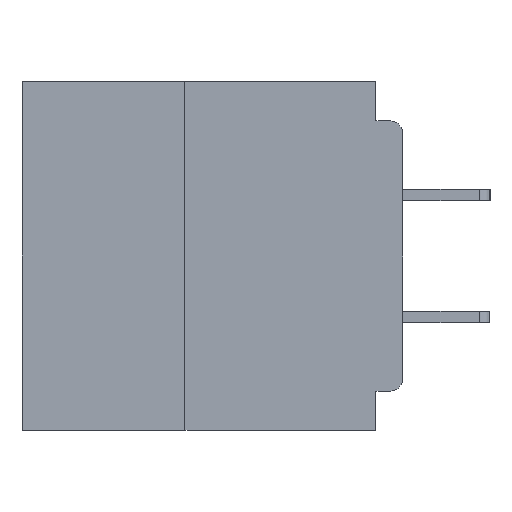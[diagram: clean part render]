
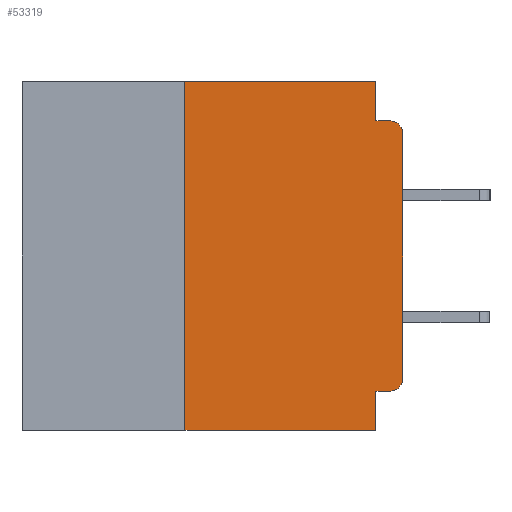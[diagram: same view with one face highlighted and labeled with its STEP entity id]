
A CAD part, left-side view. The second image highlights one B-rep face of the part: STEP entity #53319.
In plain terms, the highlighted planar face has unit normal (-1, 0, 0).
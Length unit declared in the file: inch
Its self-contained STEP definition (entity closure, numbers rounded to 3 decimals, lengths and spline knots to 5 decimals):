
#523 = VERTEX_POINT ( 'NONE', #18581 ) ;
#573 = CARTESIAN_POINT ( 'NONE',  ( 0., 0.015, -0.34 ) ) ;
#679 = VECTOR ( 'NONE', #24097, 39.37008 ) ;
#1869 = DIRECTION ( 'NONE',  ( 0., -1., 0. ) ) ;
#2103 = DIRECTION ( 'NONE',  ( 1., 0., 0. ) ) ;
#3454 = CARTESIAN_POINT ( 'NONE',  ( 0., 0.015, -0.355 ) ) ;
#3720 = ORIENTED_EDGE ( 'NONE', *, *, #36649, .F. ) ;
#3926 = EDGE_CURVE ( 'NONE', #68201, #61689, #35917, .T. ) ;
#5404 = ORIENTED_EDGE ( 'NONE', *, *, #3926, .F. ) ;
#5471 = ORIENTED_EDGE ( 'NONE', *, *, #68356, .F. ) ;
#5803 = AXIS2_PLACEMENT_3D ( 'NONE', #46922, #14716, #52354 ) ;
#6005 = DIRECTION ( 'NONE',  ( 0., 0., -1. ) ) ;
#6274 = CARTESIAN_POINT ( 'NONE',  ( 0., 0., -0.34 ) ) ;
#7348 = EDGE_CURVE ( 'NONE', #57912, #8543, #30695, .T. ) ;
#8543 = VERTEX_POINT ( 'NONE', #15496 ) ;
#9065 = VECTOR ( 'NONE', #60375, 39.37008 ) ;
#10386 = ORIENTED_EDGE ( 'NONE', *, *, #60311, .T. ) ;
#10622 = VECTOR ( 'NONE', #22715, 39.37008 ) ;
#10659 = DIRECTION ( 'NONE',  ( 0., 0., 1. ) ) ;
#11009 = CARTESIAN_POINT ( 'NONE',  ( 0., 0.031, 0. ) ) ;
#12634 = EDGE_LOOP ( 'NONE', ( #10386, #66667, #3720, #5404, #62561, #31490, #27329, #32345, #5471, #67608 ) ) ;
#13352 = AXIS2_PLACEMENT_3D ( 'NONE', #573, #38106, #6005 ) ;
#14393 = VERTEX_POINT ( 'NONE', #17084 ) ;
#14716 = DIRECTION ( 'NONE',  ( -1., 0., 0. ) ) ;
#14922 = LINE ( 'NONE', #50863, #679 ) ;
#15496 = CARTESIAN_POINT ( 'NONE',  ( 0., 0.031, -0.4 ) ) ;
#17084 = CARTESIAN_POINT ( 'NONE',  ( 0., 0., -0.06 ) ) ;
#18581 = CARTESIAN_POINT ( 'NONE',  ( 0., 0.015, -0.045 ) ) ;
#21238 = LINE ( 'NONE', #30788, #48150 ) ;
#21495 = VERTEX_POINT ( 'NONE', #29235 ) ;
#21569 = CARTESIAN_POINT ( 'NONE',  ( 0., 0.031, -0.4 ) ) ;
#21632 = CARTESIAN_POINT ( 'NONE',  ( 0., 0.031, -0.045 ) ) ;
#22715 = DIRECTION ( 'NONE',  ( 0., 1., 0. ) ) ;
#23005 = CARTESIAN_POINT ( 'NONE',  ( 0., 0.031, 0. ) ) ;
#23588 = CARTESIAN_POINT ( 'NONE',  ( 0., 0.031, -0.355 ) ) ;
#23986 = VECTOR ( 'NONE', #55055, 39.37008 ) ;
#24097 = DIRECTION ( 'NONE',  ( 0., -1., 0. ) ) ;
#26006 = VERTEX_POINT ( 'NONE', #3454 ) ;
#26617 = LINE ( 'NONE', #49504, #10622 ) ;
#27022 = DIRECTION ( 'NONE',  ( 0., 0., -1. ) ) ;
#27053 = FACE_OUTER_BOUND ( 'NONE', #12634, .T. ) ;
#27329 = ORIENTED_EDGE ( 'NONE', *, *, #68976, .T. ) ;
#29235 = CARTESIAN_POINT ( 'NONE',  ( 0., 0.25, 0. ) ) ;
#30695 = LINE ( 'NONE', #21569, #44917 ) ;
#30788 = CARTESIAN_POINT ( 'NONE',  ( 0., 0., 0. ) ) ;
#31490 = ORIENTED_EDGE ( 'NONE', *, *, #32082, .F. ) ;
#32082 = EDGE_CURVE ( 'NONE', #67657, #21495, #64169, .T. ) ;
#32345 = ORIENTED_EDGE ( 'NONE', *, *, #7348, .F. ) ;
#35253 = LINE ( 'NONE', #44806, #63828 ) ;
#35917 = LINE ( 'NONE', #23005, #9065 ) ;
#36120 = DIRECTION ( 'NONE',  ( 0., 0., 1. ) ) ;
#36649 = EDGE_CURVE ( 'NONE', #61689, #523, #35253, .T. ) ;
#37370 = EDGE_CURVE ( 'NONE', #21495, #68201, #14922, .T. ) ;
#37373 = CARTESIAN_POINT ( 'NONE',  ( 0., 0.25, -0.4 ) ) ;
#38106 = DIRECTION ( 'NONE',  ( -1., 0., 0. ) ) ;
#38196 = LINE ( 'NONE', #38793, #23986 ) ;
#38793 = CARTESIAN_POINT ( 'NONE',  ( 0., 0.437, -0.4 ) ) ;
#39615 = DIRECTION ( 'NONE',  ( 0., 0., -1. ) ) ;
#44806 = CARTESIAN_POINT ( 'NONE',  ( 0., 0., -0.045 ) ) ;
#44917 = VECTOR ( 'NONE', #27022, 39.37008 ) ;
#46922 = CARTESIAN_POINT ( 'NONE',  ( 0., 0.015, -0.06 ) ) ;
#48150 = VECTOR ( 'NONE', #36120, 39.37008 ) ;
#49147 = CARTESIAN_POINT ( 'NONE',  ( 0., 0.25, -0.4 ) ) ;
#49504 = CARTESIAN_POINT ( 'NONE',  ( 0., 0., -0.355 ) ) ;
#49901 = VECTOR ( 'NONE', #10659, 39.37008 ) ;
#50244 = PLANE ( 'NONE',  #60745 ) ;
#50863 = CARTESIAN_POINT ( 'NONE',  ( 0., 0.437, 0. ) ) ;
#51846 = EDGE_CURVE ( 'NONE', #26006, #61094, #55808, .T. ) ;
#52354 = DIRECTION ( 'NONE',  ( 0., 0., -1. ) ) ;
#53319 = ADVANCED_FACE ( 'NONE', ( #27053 ), #50244, .F. ) ;
#55055 = DIRECTION ( 'NONE',  ( 0., -1., 0. ) ) ;
#55808 = CIRCLE ( 'NONE', #13352, 0.015 ) ;
#57912 = VERTEX_POINT ( 'NONE', #23588 ) ;
#58532 = EDGE_CURVE ( 'NONE', #14393, #523, #65088, .T. ) ;
#60311 = EDGE_CURVE ( 'NONE', #61094, #14393, #21238, .T. ) ;
#60375 = DIRECTION ( 'NONE',  ( 0., 0., -1. ) ) ;
#60745 = AXIS2_PLACEMENT_3D ( 'NONE', #66390, #2103, #39615 ) ;
#61094 = VERTEX_POINT ( 'NONE', #6274 ) ;
#61689 = VERTEX_POINT ( 'NONE', #21632 ) ;
#62561 = ORIENTED_EDGE ( 'NONE', *, *, #37370, .F. ) ;
#63828 = VECTOR ( 'NONE', #1869, 39.37008 ) ;
#64169 = LINE ( 'NONE', #37373, #49901 ) ;
#65088 = CIRCLE ( 'NONE', #5803, 0.015 ) ;
#66390 = CARTESIAN_POINT ( 'NONE',  ( 0., 0.437, 0. ) ) ;
#66667 = ORIENTED_EDGE ( 'NONE', *, *, #58532, .T. ) ;
#67608 = ORIENTED_EDGE ( 'NONE', *, *, #51846, .T. ) ;
#67657 = VERTEX_POINT ( 'NONE', #49147 ) ;
#68201 = VERTEX_POINT ( 'NONE', #11009 ) ;
#68356 = EDGE_CURVE ( 'NONE', #26006, #57912, #26617, .T. ) ;
#68976 = EDGE_CURVE ( 'NONE', #67657, #8543, #38196, .T. ) ;
